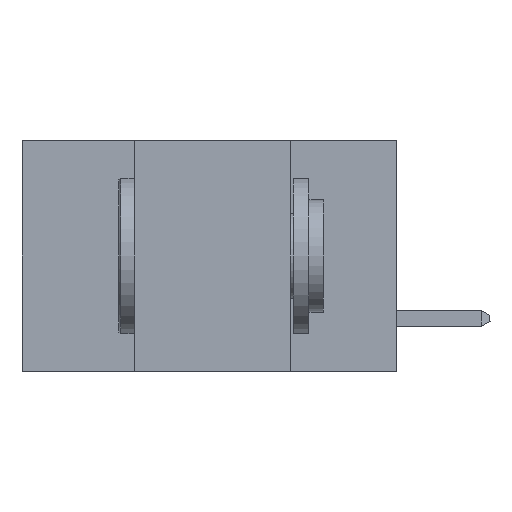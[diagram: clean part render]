
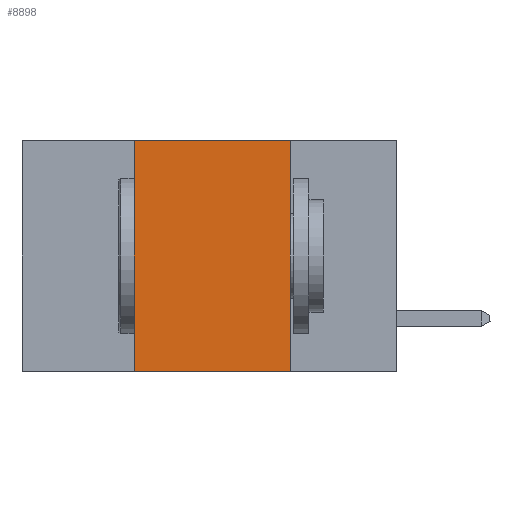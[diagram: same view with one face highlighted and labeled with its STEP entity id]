
A CAD part, left-side view. The second image highlights one B-rep face of the part: STEP entity #8898.
In plain terms, the highlighted planar face has unit normal (-1, 0, 0).
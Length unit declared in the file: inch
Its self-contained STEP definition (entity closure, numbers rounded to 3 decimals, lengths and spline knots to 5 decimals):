
#683 = LINE ( 'NONE', #9305, #4488 ) ;
#891 = CARTESIAN_POINT ( 'NONE',  ( 0., 0.42, 0. ) ) ;
#1732 = EDGE_CURVE ( 'NONE', #7392, #9863, #5709, .T. ) ;
#2366 = LINE ( 'NONE', #891, #16165 ) ;
#2384 = DIRECTION ( 'NONE',  ( 0., 0., 1. ) ) ;
#2920 = DIRECTION ( 'NONE',  ( 0., 0., -1. ) ) ;
#2923 = DIRECTION ( 'NONE',  ( 1., 0., 0. ) ) ;
#3129 = CARTESIAN_POINT ( 'NONE',  ( 0., 0.6, 0. ) ) ;
#3171 = PLANE ( 'NONE',  #15228 ) ;
#3331 = ORIENTED_EDGE ( 'NONE', *, *, #5673, .F. ) ;
#3570 = EDGE_LOOP ( 'NONE', ( #6184, #3331, #11257, #4214 ) ) ;
#4214 = ORIENTED_EDGE ( 'NONE', *, *, #1732, .T. ) ;
#4488 = VECTOR ( 'NONE', #9359, 39.37008 ) ;
#5588 = DIRECTION ( 'NONE',  ( 0., -1., 0. ) ) ;
#5673 = EDGE_CURVE ( 'NONE', #14198, #9849, #683, .T. ) ;
#5679 = EDGE_CURVE ( 'NONE', #9849, #9863, #8666, .T. ) ;
#5709 = LINE ( 'NONE', #10181, #12252 ) ;
#6184 = ORIENTED_EDGE ( 'NONE', *, *, #5679, .F. ) ;
#7392 = VERTEX_POINT ( 'NONE', #15092 ) ;
#8213 = VECTOR ( 'NONE', #17432, 39.37008 ) ;
#8666 = LINE ( 'NONE', #17258, #8213 ) ;
#8898 = ADVANCED_FACE ( 'NONE', ( #13882 ), #3171, .F. ) ;
#9305 = CARTESIAN_POINT ( 'NONE',  ( 0., 0.6, 0. ) ) ;
#9359 = DIRECTION ( 'NONE',  ( 0., -1., 0. ) ) ;
#9849 = VERTEX_POINT ( 'NONE', #12555 ) ;
#9863 = VERTEX_POINT ( 'NONE', #11282 ) ;
#10181 = CARTESIAN_POINT ( 'NONE',  ( 0., 0.6, -0.37 ) ) ;
#10564 = CARTESIAN_POINT ( 'NONE',  ( 0., 0.42, 0. ) ) ;
#11257 = ORIENTED_EDGE ( 'NONE', *, *, #14300, .F. ) ;
#11282 = CARTESIAN_POINT ( 'NONE',  ( 0., 0.17, -0.37 ) ) ;
#12252 = VECTOR ( 'NONE', #5588, 39.37008 ) ;
#12555 = CARTESIAN_POINT ( 'NONE',  ( 0., 0.17, 0. ) ) ;
#13882 = FACE_OUTER_BOUND ( 'NONE', #3570, .T. ) ;
#14198 = VERTEX_POINT ( 'NONE', #10564 ) ;
#14300 = EDGE_CURVE ( 'NONE', #7392, #14198, #2366, .T. ) ;
#15092 = CARTESIAN_POINT ( 'NONE',  ( 0., 0.42, -0.37 ) ) ;
#15228 = AXIS2_PLACEMENT_3D ( 'NONE', #3129, #2923, #2920 ) ;
#16165 = VECTOR ( 'NONE', #2384, 39.37008 ) ;
#17258 = CARTESIAN_POINT ( 'NONE',  ( 0., 0.17, 0. ) ) ;
#17432 = DIRECTION ( 'NONE',  ( 0., 0., -1. ) ) ;
